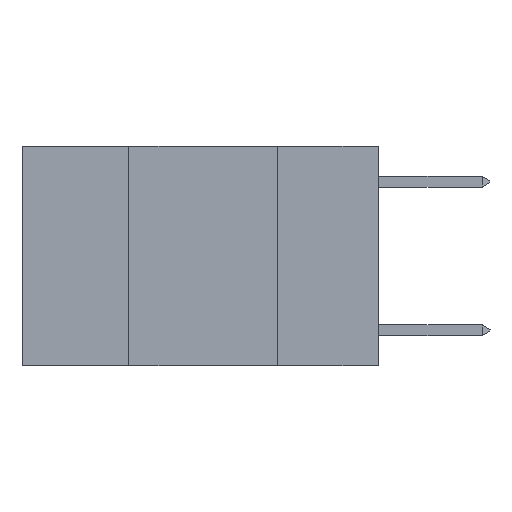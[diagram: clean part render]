
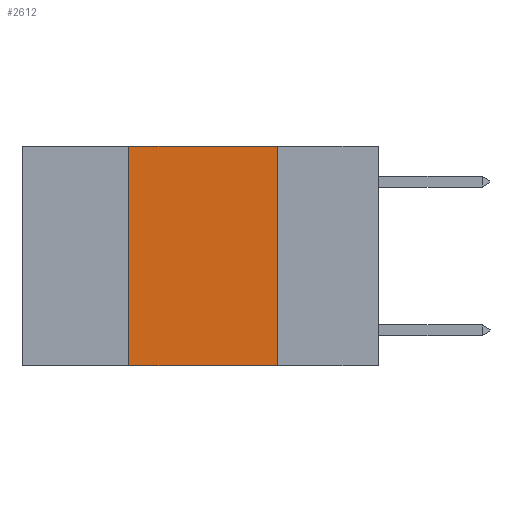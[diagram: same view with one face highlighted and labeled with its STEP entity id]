
A CAD part, left-side view. The second image highlights one B-rep face of the part: STEP entity #2612.
In plain terms, the highlighted planar face has unit normal (-1, 0, 0).
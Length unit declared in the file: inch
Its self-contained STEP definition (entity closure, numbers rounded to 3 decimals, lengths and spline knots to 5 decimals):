
#573 = CARTESIAN_POINT ( 'NONE',  ( 0., 0.42, 0. ) ) ;
#1144 = DIRECTION ( 'NONE',  ( 0., 0., -1. ) ) ;
#1388 = VECTOR ( 'NONE', #2241, 39.37008 ) ;
#1485 = VERTEX_POINT ( 'NONE', #3312 ) ;
#2241 = DIRECTION ( 'NONE',  ( 0., -1., 0. ) ) ;
#2510 = VECTOR ( 'NONE', #7432, 39.37008 ) ;
#2612 = ADVANCED_FACE ( 'NONE', ( #10710 ), #15830, .F. ) ;
#2770 = ORIENTED_EDGE ( 'NONE', *, *, #12549, .F. ) ;
#3312 = CARTESIAN_POINT ( 'NONE',  ( 0., 0.17, 0. ) ) ;
#3357 = DIRECTION ( 'NONE',  ( 1., 0., 0. ) ) ;
#3554 = ORIENTED_EDGE ( 'NONE', *, *, #5373, .F. ) ;
#4038 = DIRECTION ( 'NONE',  ( 0., 0., -1. ) ) ;
#4432 = VERTEX_POINT ( 'NONE', #12529 ) ;
#5251 = CARTESIAN_POINT ( 'NONE',  ( 0., 0.17, 0. ) ) ;
#5358 = VECTOR ( 'NONE', #6459, 39.37008 ) ;
#5373 = EDGE_CURVE ( 'NONE', #1485, #8328, #6058, .T. ) ;
#6058 = LINE ( 'NONE', #5251, #15815 ) ;
#6459 = DIRECTION ( 'NONE',  ( 0., -1., 0. ) ) ;
#7432 = DIRECTION ( 'NONE',  ( 0., 0., 1. ) ) ;
#8328 = VERTEX_POINT ( 'NONE', #10939 ) ;
#8608 = LINE ( 'NONE', #15624, #1388 ) ;
#10705 = VERTEX_POINT ( 'NONE', #16611 ) ;
#10710 = FACE_OUTER_BOUND ( 'NONE', #15013, .T. ) ;
#10939 = CARTESIAN_POINT ( 'NONE',  ( 0., 0.17, -0.37 ) ) ;
#12281 = CARTESIAN_POINT ( 'NONE',  ( 0., 0.6, 0. ) ) ;
#12529 = CARTESIAN_POINT ( 'NONE',  ( 0., 0.42, 0. ) ) ;
#12549 = EDGE_CURVE ( 'NONE', #10705, #4432, #16694, .T. ) ;
#13115 = ORIENTED_EDGE ( 'NONE', *, *, #16509, .T. ) ;
#13153 = CARTESIAN_POINT ( 'NONE',  ( 0., 0.6, -0.37 ) ) ;
#13759 = EDGE_CURVE ( 'NONE', #4432, #1485, #8608, .T. ) ;
#14510 = ORIENTED_EDGE ( 'NONE', *, *, #13759, .F. ) ;
#15013 = EDGE_LOOP ( 'NONE', ( #3554, #14510, #2770, #13115 ) ) ;
#15254 = AXIS2_PLACEMENT_3D ( 'NONE', #12281, #3357, #4038 ) ;
#15624 = CARTESIAN_POINT ( 'NONE',  ( 0., 0.6, 0. ) ) ;
#15815 = VECTOR ( 'NONE', #1144, 39.37008 ) ;
#15830 = PLANE ( 'NONE',  #15254 ) ;
#15973 = LINE ( 'NONE', #13153, #5358 ) ;
#16509 = EDGE_CURVE ( 'NONE', #10705, #8328, #15973, .T. ) ;
#16611 = CARTESIAN_POINT ( 'NONE',  ( 0., 0.42, -0.37 ) ) ;
#16694 = LINE ( 'NONE', #573, #2510 ) ;
